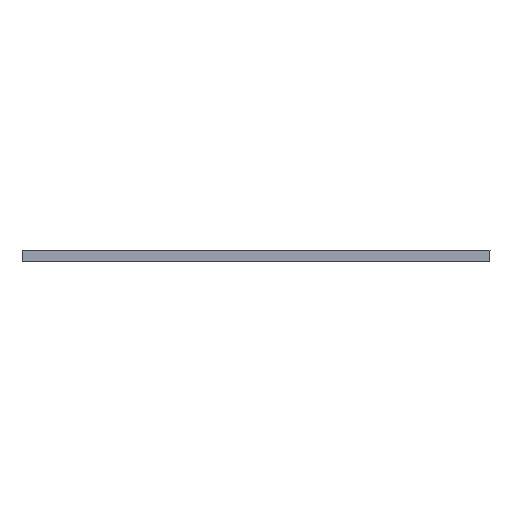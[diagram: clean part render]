
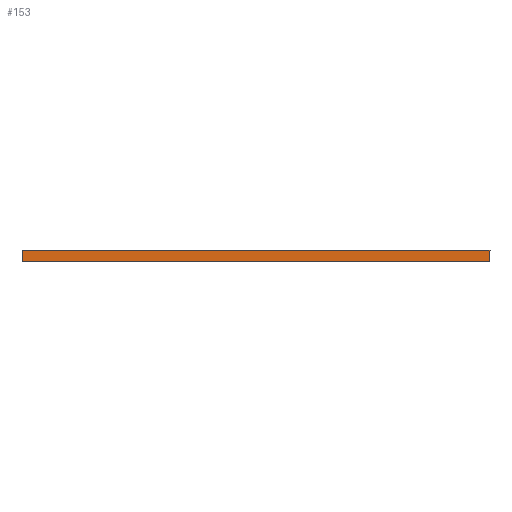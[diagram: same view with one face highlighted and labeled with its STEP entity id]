
A CAD part, left-side view. The second image highlights one B-rep face of the part: STEP entity #153.
In plain terms, the highlighted planar face has unit normal (-1, 0, 0).
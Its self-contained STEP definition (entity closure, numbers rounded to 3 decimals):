
#153 = ADVANCED_FACE ( 'NONE', ( #27008 ), #34563, .F. ) ;
#2676 = LINE ( 'NONE', #30798, #21274 ) ;
#3826 = LINE ( 'NONE', #7233, #12582 ) ;
#4398 = VERTEX_POINT ( 'NONE', #22048 ) ;
#7233 = CARTESIAN_POINT ( 'NONE',  ( -22.811, 20.5, 22.127 ) ) ;
#7817 = EDGE_LOOP ( 'NONE', ( #33038, #17587, #11317, #30346 ) ) ;
#9545 = EDGE_CURVE ( 'NONE', #33268, #27954, #3826, .T. ) ;
#11317 = ORIENTED_EDGE ( 'NONE', *, *, #9545, .F. ) ;
#12582 = VECTOR ( 'NONE', #22357, 1000. ) ;
#12804 = CARTESIAN_POINT ( 'NONE',  ( -22.811, -19.5, 22.127 ) ) ;
#13947 = CARTESIAN_POINT ( 'NONE',  ( -22.811, -19.5, 22.127 ) ) ;
#16702 = EDGE_CURVE ( 'NONE', #27954, #4398, #19171, .T. ) ;
#17587 = ORIENTED_EDGE ( 'NONE', *, *, #16702, .F. ) ;
#17677 = DIRECTION ( 'NONE',  ( 0., 0., -1. ) ) ;
#19171 = LINE ( 'NONE', #13947, #27896 ) ;
#19769 = DIRECTION ( 'NONE',  ( 0., 1., 0. ) ) ;
#21274 = VECTOR ( 'NONE', #34514, 1000. ) ;
#21577 = CARTESIAN_POINT ( 'NONE',  ( -22.811, 20.5, 21.127 ) ) ;
#22048 = CARTESIAN_POINT ( 'NONE',  ( -22.811, -19.5, 21.127 ) ) ;
#22357 = DIRECTION ( 'NONE',  ( 0., -1., 0. ) ) ;
#24874 = DIRECTION ( 'NONE',  ( 0., -1., 0. ) ) ;
#25198 = VERTEX_POINT ( 'NONE', #21577 ) ;
#27008 = FACE_OUTER_BOUND ( 'NONE', #7817, .T. ) ;
#27896 = VECTOR ( 'NONE', #17677, 1000. ) ;
#27954 = VERTEX_POINT ( 'NONE', #12804 ) ;
#28608 = CARTESIAN_POINT ( 'NONE',  ( -22.811, 20.5, 21.127 ) ) ;
#29072 = EDGE_CURVE ( 'NONE', #25198, #4398, #36135, .T. ) ;
#30346 = ORIENTED_EDGE ( 'NONE', *, *, #42040, .T. ) ;
#30798 = CARTESIAN_POINT ( 'NONE',  ( -22.811, 20.5, 22.127 ) ) ;
#32644 = CARTESIAN_POINT ( 'NONE',  ( -22.811, 20.5, 22.127 ) ) ;
#33038 = ORIENTED_EDGE ( 'NONE', *, *, #29072, .T. ) ;
#33268 = VERTEX_POINT ( 'NONE', #32644 ) ;
#33869 = AXIS2_PLACEMENT_3D ( 'NONE', #45644, #42048, #19769 ) ;
#34514 = DIRECTION ( 'NONE',  ( 0., 0., -1. ) ) ;
#34563 = PLANE ( 'NONE',  #33869 ) ;
#36135 = LINE ( 'NONE', #28608, #44881 ) ;
#42040 = EDGE_CURVE ( 'NONE', #33268, #25198, #2676, .T. ) ;
#42048 = DIRECTION ( 'NONE',  ( 1., 0., 0. ) ) ;
#44881 = VECTOR ( 'NONE', #24874, 1000. ) ;
#45644 = CARTESIAN_POINT ( 'NONE',  ( -22.811, 20.5, 22.127 ) ) ;
